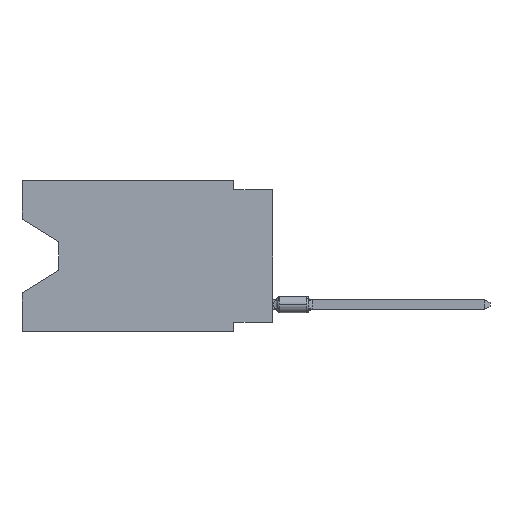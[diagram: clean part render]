
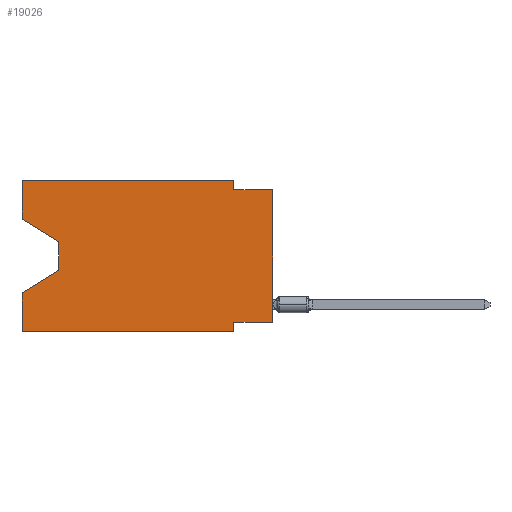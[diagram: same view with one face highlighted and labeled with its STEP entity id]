
A CAD part, left-side view. The second image highlights one B-rep face of the part: STEP entity #19026.
In plain terms, the highlighted planar face has unit normal (-1, 0, 0).
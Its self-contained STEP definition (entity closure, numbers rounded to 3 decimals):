
#178 = VECTOR ( 'NONE', #18956, 1000. ) ;
#255 = CARTESIAN_POINT ( 'NONE',  ( 0., 2.54, -9.271 ) ) ;
#304 = PLANE ( 'NONE',  #5617 ) ;
#721 = DIRECTION ( 'NONE',  ( 0., -1., 0. ) ) ;
#874 = VECTOR ( 'NONE', #11330, 1000. ) ;
#1057 = VECTOR ( 'NONE', #14623, 1000. ) ;
#1184 = EDGE_CURVE ( 'NONE', #2380, #17571, #16644, .T. ) ;
#1266 = DIRECTION ( 'NONE',  ( 0., -1., 0. ) ) ;
#1441 = VERTEX_POINT ( 'NONE', #13310 ) ;
#1531 = DIRECTION ( 'NONE',  ( 0., 0.855, -0.519 ) ) ;
#2380 = VERTEX_POINT ( 'NONE', #5987 ) ;
#2439 = CARTESIAN_POINT ( 'NONE',  ( 0., 13.97, -5.893 ) ) ;
#2748 = CARTESIAN_POINT ( 'NONE',  ( 0., 0., -0.635 ) ) ;
#2875 = VERTEX_POINT ( 'NONE', #9061 ) ;
#3023 = DIRECTION ( 'NONE',  ( 0., 0., 1. ) ) ;
#3298 = ORIENTED_EDGE ( 'NONE', *, *, #19230, .F. ) ;
#3376 = CARTESIAN_POINT ( 'NONE',  ( 0., 16.383, -7.36 ) ) ;
#3400 = EDGE_CURVE ( 'NONE', #18021, #7837, #5380, .T. ) ;
#3530 = EDGE_CURVE ( 'NONE', #14567, #3811, #8750, .T. ) ;
#3576 = VECTOR ( 'NONE', #16473, 1000. ) ;
#3808 = ORIENTED_EDGE ( 'NONE', *, *, #1184, .F. ) ;
#3809 = ORIENTED_EDGE ( 'NONE', *, *, #5983, .T. ) ;
#3811 = VERTEX_POINT ( 'NONE', #10130 ) ;
#4201 = ORIENTED_EDGE ( 'NONE', *, *, #6857, .F. ) ;
#4347 = CARTESIAN_POINT ( 'NONE',  ( 0., 16.383, 0. ) ) ;
#4864 = DIRECTION ( 'NONE',  ( 0., 0., -1. ) ) ;
#4985 = DIRECTION ( 'NONE',  ( 0., -1., 0. ) ) ;
#5048 = LINE ( 'NONE', #17181, #18985 ) ;
#5241 = ORIENTED_EDGE ( 'NONE', *, *, #15005, .F. ) ;
#5380 = LINE ( 'NONE', #14342, #7772 ) ;
#5516 = EDGE_CURVE ( 'NONE', #9104, #14149, #18120, .T. ) ;
#5537 = VECTOR ( 'NONE', #4985, 1000. ) ;
#5617 = AXIS2_PLACEMENT_3D ( 'NONE', #6352, #16909, #14020 ) ;
#5983 = EDGE_CURVE ( 'NONE', #14363, #9104, #7743, .T. ) ;
#5987 = CARTESIAN_POINT ( 'NONE',  ( 0., 16.383, -2.546 ) ) ;
#6216 = VECTOR ( 'NONE', #1266, 1000. ) ;
#6352 = CARTESIAN_POINT ( 'NONE',  ( 0., 16.383, 0. ) ) ;
#6414 = CARTESIAN_POINT ( 'NONE',  ( 0., 16.383, -2.546 ) ) ;
#6857 = EDGE_CURVE ( 'NONE', #2875, #18021, #17907, .T. ) ;
#7224 = LINE ( 'NONE', #17587, #6216 ) ;
#7227 = LINE ( 'NONE', #4347, #18249 ) ;
#7360 = CARTESIAN_POINT ( 'NONE',  ( 0., 13.97, -5.893 ) ) ;
#7743 = LINE ( 'NONE', #7945, #8029 ) ;
#7772 = VECTOR ( 'NONE', #721, 1000. ) ;
#7837 = VERTEX_POINT ( 'NONE', #2748 ) ;
#7945 = CARTESIAN_POINT ( 'NONE',  ( 0., 13.97, -4.013 ) ) ;
#8029 = VECTOR ( 'NONE', #4864, 1000. ) ;
#8530 = LINE ( 'NONE', #17507, #874 ) ;
#8634 = EDGE_CURVE ( 'NONE', #1441, #7837, #11870, .T. ) ;
#8648 = VECTOR ( 'NONE', #1531, 1000. ) ;
#8750 = LINE ( 'NONE', #14835, #5537 ) ;
#8976 = ORIENTED_EDGE ( 'NONE', *, *, #3530, .T. ) ;
#9061 = CARTESIAN_POINT ( 'NONE',  ( 0., 2.54, 0. ) ) ;
#9104 = VERTEX_POINT ( 'NONE', #2439 ) ;
#10130 = CARTESIAN_POINT ( 'NONE',  ( 0., 2.54, -9.906 ) ) ;
#10338 = CARTESIAN_POINT ( 'NONE',  ( 0., 16.383, -9.906 ) ) ;
#10401 = CARTESIAN_POINT ( 'NONE',  ( 0., 0., 0. ) ) ;
#10564 = EDGE_LOOP ( 'NONE', ( #17454, #3809, #19148, #5241, #8976, #3298, #17827, #12019, #18495, #4201, #15806, #3808 ) ) ;
#10915 = EDGE_CURVE ( 'NONE', #2380, #14363, #12878, .T. ) ;
#11330 = DIRECTION ( 'NONE',  ( 0., 0., -1. ) ) ;
#11438 = CARTESIAN_POINT ( 'NONE',  ( 0., 2.54, 0. ) ) ;
#11870 = LINE ( 'NONE', #10401, #3576 ) ;
#11909 = CARTESIAN_POINT ( 'NONE',  ( 0., 2.54, -0.635 ) ) ;
#12019 = ORIENTED_EDGE ( 'NONE', *, *, #8634, .T. ) ;
#12178 = VECTOR ( 'NONE', #3023, 1000. ) ;
#12222 = FACE_OUTER_BOUND ( 'NONE', #10564, .T. ) ;
#12878 = LINE ( 'NONE', #6414, #178 ) ;
#13310 = CARTESIAN_POINT ( 'NONE',  ( 0., 0., -9.271 ) ) ;
#14020 = DIRECTION ( 'NONE',  ( 0., 0., -1. ) ) ;
#14149 = VERTEX_POINT ( 'NONE', #3376 ) ;
#14247 = CARTESIAN_POINT ( 'NONE',  ( 0., 16.383, 0. ) ) ;
#14342 = CARTESIAN_POINT ( 'NONE',  ( 0., 0., -0.635 ) ) ;
#14363 = VERTEX_POINT ( 'NONE', #16926 ) ;
#14567 = VERTEX_POINT ( 'NONE', #10338 ) ;
#14623 = DIRECTION ( 'NONE',  ( 0., 0., -1. ) ) ;
#14835 = CARTESIAN_POINT ( 'NONE',  ( 0., 16.383, -9.906 ) ) ;
#15005 = EDGE_CURVE ( 'NONE', #14567, #14149, #7227, .T. ) ;
#15806 = ORIENTED_EDGE ( 'NONE', *, *, #16434, .F. ) ;
#16434 = EDGE_CURVE ( 'NONE', #17571, #2875, #7224, .T. ) ;
#16473 = DIRECTION ( 'NONE',  ( 0., 0., 1. ) ) ;
#16644 = LINE ( 'NONE', #17056, #12178 ) ;
#16909 = DIRECTION ( 'NONE',  ( 1., 0., 0. ) ) ;
#16926 = CARTESIAN_POINT ( 'NONE',  ( 0., 13.97, -4.013 ) ) ;
#17056 = CARTESIAN_POINT ( 'NONE',  ( 0., 16.383, 0. ) ) ;
#17069 = VERTEX_POINT ( 'NONE', #255 ) ;
#17181 = CARTESIAN_POINT ( 'NONE',  ( 0., 0., -9.271 ) ) ;
#17454 = ORIENTED_EDGE ( 'NONE', *, *, #10915, .T. ) ;
#17479 = DIRECTION ( 'NONE',  ( 0., 1., 0. ) ) ;
#17507 = CARTESIAN_POINT ( 'NONE',  ( 0., 2.54, -9.906 ) ) ;
#17571 = VERTEX_POINT ( 'NONE', #14247 ) ;
#17587 = CARTESIAN_POINT ( 'NONE',  ( 0., 16.383, 0. ) ) ;
#17693 = DIRECTION ( 'NONE',  ( 0., 0., 1. ) ) ;
#17827 = ORIENTED_EDGE ( 'NONE', *, *, #18344, .F. ) ;
#17907 = LINE ( 'NONE', #11438, #1057 ) ;
#18021 = VERTEX_POINT ( 'NONE', #11909 ) ;
#18120 = LINE ( 'NONE', #7360, #8648 ) ;
#18249 = VECTOR ( 'NONE', #17693, 1000. ) ;
#18344 = EDGE_CURVE ( 'NONE', #1441, #17069, #5048, .T. ) ;
#18495 = ORIENTED_EDGE ( 'NONE', *, *, #3400, .F. ) ;
#18956 = DIRECTION ( 'NONE',  ( 0., -0.855, -0.519 ) ) ;
#18985 = VECTOR ( 'NONE', #17479, 1000. ) ;
#19026 = ADVANCED_FACE ( 'NONE', ( #12222 ), #304, .F. ) ;
#19148 = ORIENTED_EDGE ( 'NONE', *, *, #5516, .T. ) ;
#19230 = EDGE_CURVE ( 'NONE', #17069, #3811, #8530, .T. ) ;
